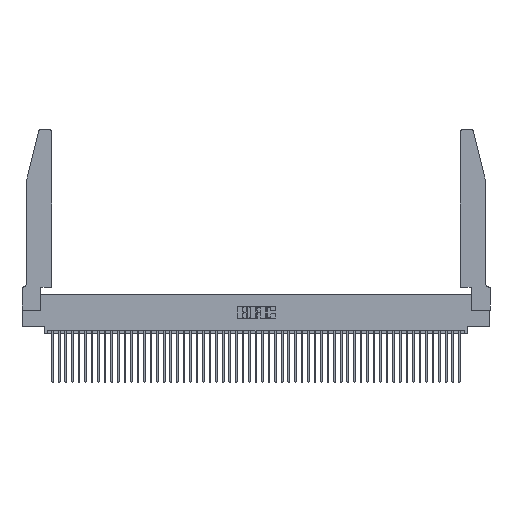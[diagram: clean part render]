
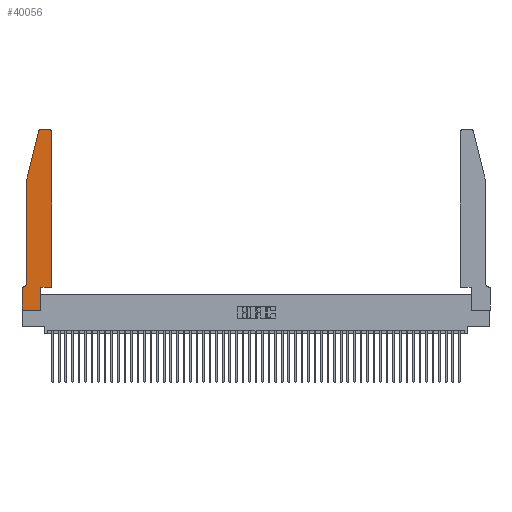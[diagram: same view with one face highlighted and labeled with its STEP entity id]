
A CAD part, top view. The second image highlights one B-rep face of the part: STEP entity #40056.
In plain terms, the highlighted planar face has unit normal (0, 0, 1).
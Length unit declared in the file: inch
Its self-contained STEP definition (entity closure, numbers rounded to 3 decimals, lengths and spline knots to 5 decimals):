
#5 = LINE ( 'NONE', #49755, #4424 ) ;
#236 = EDGE_LOOP ( 'NONE', ( #2032, #43838, #17753, #15551, #34061, #38213, #36137, #29086, #2385, #29440, #10639, #25805 ) ) ;
#957 = VECTOR ( 'NONE', #10836, 39.37008 ) ;
#1685 = VECTOR ( 'NONE', #7057, 39.37008 ) ;
#2032 = ORIENTED_EDGE ( 'NONE', *, *, #10380, .T. ) ;
#2165 = AXIS2_PLACEMENT_3D ( 'NONE', #46017, #30355, #17703 ) ;
#2167 = CARTESIAN_POINT ( 'NONE',  ( 0.4505, 0.35, 0.37 ) ) ;
#2264 = CIRCLE ( 'NONE', #27748, 0.03 ) ;
#2385 = ORIENTED_EDGE ( 'NONE', *, *, #46487, .T. ) ;
#3245 = CARTESIAN_POINT ( 'NONE',  ( 0., 0., 0.37 ) ) ;
#3402 = CARTESIAN_POINT ( 'NONE',  ( 0.0755, 2., 0.37 ) ) ;
#3718 = DIRECTION ( 'NONE',  ( 0., -1., 0. ) ) ;
#3794 = VERTEX_POINT ( 'NONE', #18136 ) ;
#3948 = FACE_OUTER_BOUND ( 'NONE', #236, .T. ) ;
#4096 = VERTEX_POINT ( 'NONE', #39129 ) ;
#4424 = VECTOR ( 'NONE', #21392, 39.37008 ) ;
#5186 = CARTESIAN_POINT ( 'NONE',  ( 0.0055, 0.42, 0.37 ) ) ;
#5519 = DIRECTION ( 'NONE',  ( 0., 0., -1. ) ) ;
#6014 = LINE ( 'NONE', #11057, #15309 ) ;
#6277 = CARTESIAN_POINT ( 'NONE',  ( 0., 0.35, 0.37 ) ) ;
#6647 = LINE ( 'NONE', #41902, #27776 ) ;
#7057 = DIRECTION ( 'NONE',  ( -1., 0., 0. ) ) ;
#9475 = VECTOR ( 'NONE', #18500, 39.37008 ) ;
#10380 = EDGE_CURVE ( 'NONE', #35422, #41809, #41492, .T. ) ;
#10591 = EDGE_CURVE ( 'NONE', #28603, #3794, #6647, .T. ) ;
#10639 = ORIENTED_EDGE ( 'NONE', *, *, #47096, .T. ) ;
#10836 = DIRECTION ( 'NONE',  ( 0., 1., 0. ) ) ;
#11057 = CARTESIAN_POINT ( 'NONE',  ( 0.2865, 0.35, 0.37 ) ) ;
#12347 = LINE ( 'NONE', #28080, #41002 ) ;
#13783 = VECTOR ( 'NONE', #18549, 39.37008 ) ;
#15309 = VECTOR ( 'NONE', #38534, 39.37008 ) ;
#15551 = ORIENTED_EDGE ( 'NONE', *, *, #49782, .T. ) ;
#15856 = CIRCLE ( 'NONE', #2165, 0.03 ) ;
#16009 = DIRECTION ( 'NONE',  ( 1., 0., 0. ) ) ;
#17703 = DIRECTION ( 'NONE',  ( 1., 0., 0. ) ) ;
#17753 = ORIENTED_EDGE ( 'NONE', *, *, #10591, .T. ) ;
#18136 = CARTESIAN_POINT ( 'NONE',  ( 0.0755, 2., 0.37 ) ) ;
#18500 = DIRECTION ( 'NONE',  ( 1., 0., 0. ) ) ;
#18549 = DIRECTION ( 'NONE',  ( 1., 0., 0. ) ) ;
#18757 = EDGE_CURVE ( 'NONE', #46961, #29861, #43043, .T. ) ;
#19434 = CARTESIAN_POINT ( 'NONE',  ( 0.284, 2.75, 0.37 ) ) ;
#19442 = EDGE_CURVE ( 'NONE', #25080, #41336, #5, .T. ) ;
#19569 = CARTESIAN_POINT ( 'NONE',  ( 0., 0., 0.37 ) ) ;
#19726 = VERTEX_POINT ( 'NONE', #43283 ) ;
#21392 = DIRECTION ( 'NONE',  ( 0., -1., 0. ) ) ;
#21832 = CIRCLE ( 'NONE', #41147, 0.07 ) ;
#22718 = DIRECTION ( 'NONE',  ( 0., 0., 1. ) ) ;
#25080 = VERTEX_POINT ( 'NONE', #6277 ) ;
#25805 = ORIENTED_EDGE ( 'NONE', *, *, #39026, .T. ) ;
#26621 = DIRECTION ( 'NONE',  ( -0.239, -0.971, 0. ) ) ;
#27207 = CARTESIAN_POINT ( 'NONE',  ( 0.2605, 2.75, 0.37 ) ) ;
#27705 = CARTESIAN_POINT ( 'NONE',  ( 0.4505, 0.35, 0.37 ) ) ;
#27748 = AXIS2_PLACEMENT_3D ( 'NONE', #31213, #22718, #42360 ) ;
#27776 = VECTOR ( 'NONE', #26621, 39.37008 ) ;
#28080 = CARTESIAN_POINT ( 'NONE',  ( 0.0755, 0.35, 0.37 ) ) ;
#28603 = VERTEX_POINT ( 'NONE', #39580 ) ;
#29086 = ORIENTED_EDGE ( 'NONE', *, *, #31072, .T. ) ;
#29440 = ORIENTED_EDGE ( 'NONE', *, *, #18757, .T. ) ;
#29861 = VERTEX_POINT ( 'NONE', #27705 ) ;
#30355 = DIRECTION ( 'NONE',  ( 0., 0., 1. ) ) ;
#31072 = EDGE_CURVE ( 'NONE', #41336, #19726, #33669, .T. ) ;
#31213 = CARTESIAN_POINT ( 'NONE',  ( 0.284, 2.72, 0.37 ) ) ;
#32337 = CARTESIAN_POINT ( 'NONE',  ( 0., 0.35, 0.37 ) ) ;
#32787 = DIRECTION ( 'NONE',  ( -1., 0., 0. ) ) ;
#32970 = VECTOR ( 'NONE', #3718, 39.37008 ) ;
#33274 = CARTESIAN_POINT ( 'NONE',  ( 0.2865, 0.35, 0.37 ) ) ;
#33669 = LINE ( 'NONE', #3245, #13783 ) ;
#34061 = ORIENTED_EDGE ( 'NONE', *, *, #40862, .T. ) ;
#34265 = EDGE_CURVE ( 'NONE', #46611, #25080, #12347, .T. ) ;
#34778 = AXIS2_PLACEMENT_3D ( 'NONE', #32337, #47683, #16009 ) ;
#35422 = VERTEX_POINT ( 'NONE', #42498 ) ;
#35963 = PLANE ( 'NONE',  #34778 ) ;
#36137 = ORIENTED_EDGE ( 'NONE', *, *, #19442, .T. ) ;
#36763 = EDGE_CURVE ( 'NONE', #41809, #28603, #2264, .T. ) ;
#36992 = LINE ( 'NONE', #2167, #957 ) ;
#37952 = VERTEX_POINT ( 'NONE', #45923 ) ;
#38213 = ORIENTED_EDGE ( 'NONE', *, *, #34265, .T. ) ;
#38534 = DIRECTION ( 'NONE',  ( 0., 1., 0. ) ) ;
#39026 = EDGE_CURVE ( 'NONE', #4096, #35422, #15856, .T. ) ;
#39129 = CARTESIAN_POINT ( 'NONE',  ( 0.4505, 2.72, 0.37 ) ) ;
#39580 = CARTESIAN_POINT ( 'NONE',  ( 0.25487, 2.72718, 0.37 ) ) ;
#40056 = ADVANCED_FACE ( 'NONE', ( #3948 ), #35963, .T. ) ;
#40862 = EDGE_CURVE ( 'NONE', #37952, #46611, #21832, .T. ) ;
#41002 = VECTOR ( 'NONE', #47739, 39.37008 ) ;
#41147 = AXIS2_PLACEMENT_3D ( 'NONE', #5186, #5519, #32787 ) ;
#41336 = VERTEX_POINT ( 'NONE', #19569 ) ;
#41492 = LINE ( 'NONE', #27207, #1685 ) ;
#41809 = VERTEX_POINT ( 'NONE', #19434 ) ;
#41902 = CARTESIAN_POINT ( 'NONE',  ( 0.0755, 2., 0.37 ) ) ;
#41966 = CARTESIAN_POINT ( 'NONE',  ( 0.4505, 0.35, 0.37 ) ) ;
#42360 = DIRECTION ( 'NONE',  ( 1., 0., 0. ) ) ;
#42498 = CARTESIAN_POINT ( 'NONE',  ( 0.4205, 2.75, 0.37 ) ) ;
#43043 = LINE ( 'NONE', #41966, #9475 ) ;
#43283 = CARTESIAN_POINT ( 'NONE',  ( 0.2865, 0., 0.37 ) ) ;
#43838 = ORIENTED_EDGE ( 'NONE', *, *, #36763, .T. ) ;
#43910 = CARTESIAN_POINT ( 'NONE',  ( 0.0055, 0.35, 0.37 ) ) ;
#44807 = LINE ( 'NONE', #3402, #32970 ) ;
#45923 = CARTESIAN_POINT ( 'NONE',  ( 0.0755, 0.42, 0.37 ) ) ;
#46017 = CARTESIAN_POINT ( 'NONE',  ( 0.4205, 2.72, 0.37 ) ) ;
#46487 = EDGE_CURVE ( 'NONE', #19726, #46961, #6014, .T. ) ;
#46611 = VERTEX_POINT ( 'NONE', #43910 ) ;
#46961 = VERTEX_POINT ( 'NONE', #33274 ) ;
#47096 = EDGE_CURVE ( 'NONE', #29861, #4096, #36992, .T. ) ;
#47683 = DIRECTION ( 'NONE',  ( 0., 0., 1. ) ) ;
#47739 = DIRECTION ( 'NONE',  ( -1., 0., 0. ) ) ;
#49755 = CARTESIAN_POINT ( 'NONE',  ( 0., 0., 0.37 ) ) ;
#49782 = EDGE_CURVE ( 'NONE', #3794, #37952, #44807, .T. ) ;
